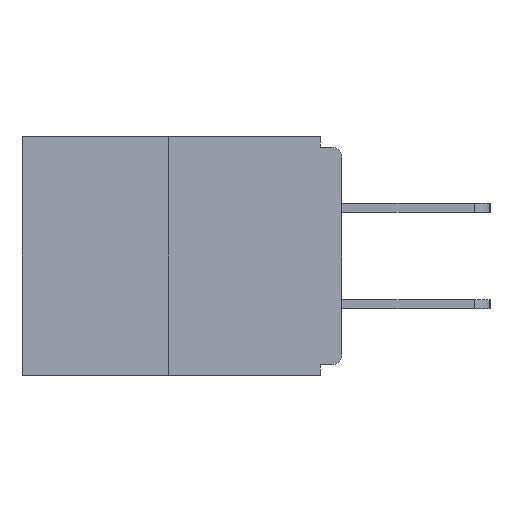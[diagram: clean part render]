
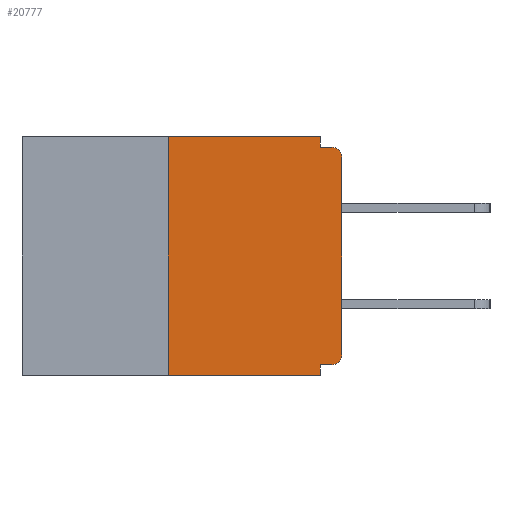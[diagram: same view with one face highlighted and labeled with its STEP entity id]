
A CAD part, left-side view. The second image highlights one B-rep face of the part: STEP entity #20777.
In plain terms, the highlighted planar face has unit normal (-1, 0, 0).
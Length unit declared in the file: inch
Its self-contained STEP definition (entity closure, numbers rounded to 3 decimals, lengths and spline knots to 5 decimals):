
#289 = FACE_OUTER_BOUND ( 'NONE', #5849, .T. ) ;
#2254 = EDGE_CURVE ( 'NONE', #15946, #15461, #7659, .T. ) ;
#2730 = CARTESIAN_POINT ( 'NONE',  ( 0., 0.25, -0.343 ) ) ;
#3175 = VECTOR ( 'NONE', #24174, 39.37008 ) ;
#3177 = EDGE_CURVE ( 'NONE', #3194, #18381, #11607, .T. ) ;
#3194 = VERTEX_POINT ( 'NONE', #9168 ) ;
#3588 = VECTOR ( 'NONE', #5961, 39.37008 ) ;
#4003 = CIRCLE ( 'NONE', #9960, 0.015 ) ;
#4079 = VERTEX_POINT ( 'NONE', #15621 ) ;
#4403 = VECTOR ( 'NONE', #19428, 39.37008 ) ;
#4876 = VECTOR ( 'NONE', #12025, 39.37008 ) ;
#5246 = EDGE_CURVE ( 'NONE', #19550, #7342, #10908, .T. ) ;
#5318 = LINE ( 'NONE', #20192, #3175 ) ;
#5591 = CARTESIAN_POINT ( 'NONE',  ( 0., 0.031, 0. ) ) ;
#5849 = EDGE_LOOP ( 'NONE', ( #24313, #25416, #13107, #9395, #10184, #9625, #9441, #8828, #6310, #22700 ) ) ;
#5961 = DIRECTION ( 'NONE',  ( 0., -1., 0. ) ) ;
#6127 = EDGE_CURVE ( 'NONE', #15461, #16067, #5318, .T. ) ;
#6190 = DIRECTION ( 'NONE',  ( 0., 0., -1. ) ) ;
#6310 = ORIENTED_EDGE ( 'NONE', *, *, #3177, .F. ) ;
#6471 = PLANE ( 'NONE',  #20823 ) ;
#6625 = CARTESIAN_POINT ( 'NONE',  ( 0., 0.46, 0. ) ) ;
#6965 = DIRECTION ( 'NONE',  ( 0., -1., 0. ) ) ;
#7342 = VERTEX_POINT ( 'NONE', #13487 ) ;
#7456 = LINE ( 'NONE', #20755, #18606 ) ;
#7476 = CARTESIAN_POINT ( 'NONE',  ( 0., 0., -0.313 ) ) ;
#7659 = LINE ( 'NONE', #21493, #4876 ) ;
#8513 = VECTOR ( 'NONE', #14878, 39.37008 ) ;
#8828 = ORIENTED_EDGE ( 'NONE', *, *, #15196, .T. ) ;
#9168 = CARTESIAN_POINT ( 'NONE',  ( 0., 0.031, -0.015 ) ) ;
#9202 = CARTESIAN_POINT ( 'NONE',  ( 0., 0.031, -0.343 ) ) ;
#9395 = ORIENTED_EDGE ( 'NONE', *, *, #6127, .F. ) ;
#9441 = ORIENTED_EDGE ( 'NONE', *, *, #23586, .T. ) ;
#9625 = ORIENTED_EDGE ( 'NONE', *, *, #13082, .T. ) ;
#9960 = AXIS2_PLACEMENT_3D ( 'NONE', #15843, #11944, #6190 ) ;
#10086 = EDGE_CURVE ( 'NONE', #19550, #16067, #22475, .T. ) ;
#10184 = ORIENTED_EDGE ( 'NONE', *, *, #2254, .F. ) ;
#10908 = LINE ( 'NONE', #13950, #25147 ) ;
#11607 = LINE ( 'NONE', #20781, #8513 ) ;
#11944 = DIRECTION ( 'NONE',  ( -1., 0., 0. ) ) ;
#12025 = DIRECTION ( 'NONE',  ( 0., 1., 0. ) ) ;
#12719 = LINE ( 'NONE', #5591, #4403 ) ;
#12761 = CARTESIAN_POINT ( 'NONE',  ( 0., 0.46, 0. ) ) ;
#13082 = EDGE_CURVE ( 'NONE', #15946, #19905, #13693, .T. ) ;
#13107 = ORIENTED_EDGE ( 'NONE', *, *, #10086, .T. ) ;
#13310 = DIRECTION ( 'NONE',  ( 0., 0., -1. ) ) ;
#13487 = CARTESIAN_POINT ( 'NONE',  ( 0., 0.25, 0. ) ) ;
#13693 = CIRCLE ( 'NONE', #22356, 0.015 ) ;
#13950 = CARTESIAN_POINT ( 'NONE',  ( 0., 0.25, 0. ) ) ;
#14029 = DIRECTION ( 'NONE',  ( 0., 0., 1. ) ) ;
#14878 = DIRECTION ( 'NONE',  ( 0., -1., 0. ) ) ;
#15196 = EDGE_CURVE ( 'NONE', #23617, #18381, #4003, .T. ) ;
#15461 = VERTEX_POINT ( 'NONE', #23102 ) ;
#15621 = CARTESIAN_POINT ( 'NONE',  ( 0., 0.031, 0. ) ) ;
#15843 = CARTESIAN_POINT ( 'NONE',  ( 0., 0.015, -0.03 ) ) ;
#15946 = VERTEX_POINT ( 'NONE', #16658 ) ;
#16067 = VERTEX_POINT ( 'NONE', #9202 ) ;
#16658 = CARTESIAN_POINT ( 'NONE',  ( 0., 0.015, -0.328 ) ) ;
#16899 = EDGE_CURVE ( 'NONE', #7342, #4079, #19666, .T. ) ;
#18381 = VERTEX_POINT ( 'NONE', #22390 ) ;
#18529 = DIRECTION ( 'NONE',  ( 0., 0., 1. ) ) ;
#18606 = VECTOR ( 'NONE', #18529, 39.37008 ) ;
#18618 = EDGE_CURVE ( 'NONE', #4079, #3194, #12719, .T. ) ;
#18666 = DIRECTION ( 'NONE',  ( 1., 0., 0. ) ) ;
#19428 = DIRECTION ( 'NONE',  ( 0., 0., -1. ) ) ;
#19493 = CARTESIAN_POINT ( 'NONE',  ( 0., 0.015, -0.313 ) ) ;
#19550 = VERTEX_POINT ( 'NONE', #2730 ) ;
#19666 = LINE ( 'NONE', #6625, #23687 ) ;
#19905 = VERTEX_POINT ( 'NONE', #7476 ) ;
#20192 = CARTESIAN_POINT ( 'NONE',  ( 0., 0.031, -0.343 ) ) ;
#20671 = CARTESIAN_POINT ( 'NONE',  ( 0., 0., -0.03 ) ) ;
#20755 = CARTESIAN_POINT ( 'NONE',  ( 0., 0., 0. ) ) ;
#20777 = ADVANCED_FACE ( 'NONE', ( #289 ), #6471, .F. ) ;
#20781 = CARTESIAN_POINT ( 'NONE',  ( 0., 0., -0.015 ) ) ;
#20823 = AXIS2_PLACEMENT_3D ( 'NONE', #12761, #18666, #24292 ) ;
#21493 = CARTESIAN_POINT ( 'NONE',  ( 0., 0., -0.328 ) ) ;
#22356 = AXIS2_PLACEMENT_3D ( 'NONE', #19493, #25525, #13310 ) ;
#22390 = CARTESIAN_POINT ( 'NONE',  ( 0., 0.015, -0.015 ) ) ;
#22475 = LINE ( 'NONE', #23846, #3588 ) ;
#22700 = ORIENTED_EDGE ( 'NONE', *, *, #18618, .F. ) ;
#23102 = CARTESIAN_POINT ( 'NONE',  ( 0., 0.031, -0.328 ) ) ;
#23586 = EDGE_CURVE ( 'NONE', #19905, #23617, #7456, .T. ) ;
#23617 = VERTEX_POINT ( 'NONE', #20671 ) ;
#23687 = VECTOR ( 'NONE', #6965, 39.37008 ) ;
#23846 = CARTESIAN_POINT ( 'NONE',  ( 0., 0.46, -0.343 ) ) ;
#24174 = DIRECTION ( 'NONE',  ( 0., 0., -1. ) ) ;
#24292 = DIRECTION ( 'NONE',  ( 0., 0., -1. ) ) ;
#24313 = ORIENTED_EDGE ( 'NONE', *, *, #16899, .F. ) ;
#25147 = VECTOR ( 'NONE', #14029, 39.37008 ) ;
#25416 = ORIENTED_EDGE ( 'NONE', *, *, #5246, .F. ) ;
#25525 = DIRECTION ( 'NONE',  ( -1., 0., 0. ) ) ;
